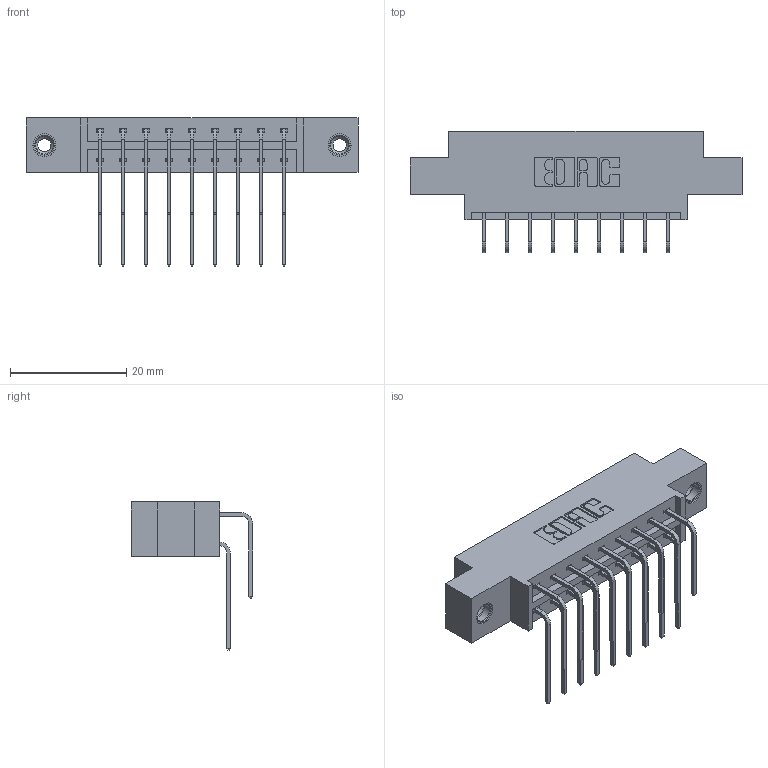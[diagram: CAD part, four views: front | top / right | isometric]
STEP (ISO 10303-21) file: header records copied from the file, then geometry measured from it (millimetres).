
FILE_DESCRIPTION (( 'STEP AP203' ), '1' );
FILE_NAME ('833-018-559-808.STEP', '2020-05-31T23:36:53', ( '' ), ( '' ), 'SwSTEP 2.0', 'SolidWorks 2020', '' );
FILE_SCHEMA (( 'CONFIG_CONTROL_DESIGN' ));
Length unit declared in the file: inch
Products named in the file (5): 833-018-559-808; 345-292-001_558 559 Tail - 1; 833 Part_Offset - .156 Dia - TI; 345-250-001_345-250-003-102; 345-292-001_559 Tail - 2
Assembly tree (21 placements, depth 2):
  833-018-559-808
    833 Part_Offset - .156 Dia - TI
    345-292-001_558 559 Tail - 1  x9
    345-292-001_559 Tail - 2  x9
    345-250-001_345-250-003-102  x2
Bounding box: 57.2 x 20.9 x 25.53 mm (x, y, z)
Volume: 5400.8 mm3; surface area: 6790.3 mm2
Topology: 21 solids, 21 shells, 1150 faces, 3357 edges, 2206 vertices
Faces by surface type: plane 790, cylinder 344, cone 12, torus 4
Entity records: 13160 total; most frequent: CARTESIAN_POINT 2256, ORIENTED_EDGE 2134, DIRECTION 1997, EDGE_CURVE 1067, LINE 879, VECTOR 879, VERTEX_POINT 704, AXIS2_PLACEMENT_3D 559
